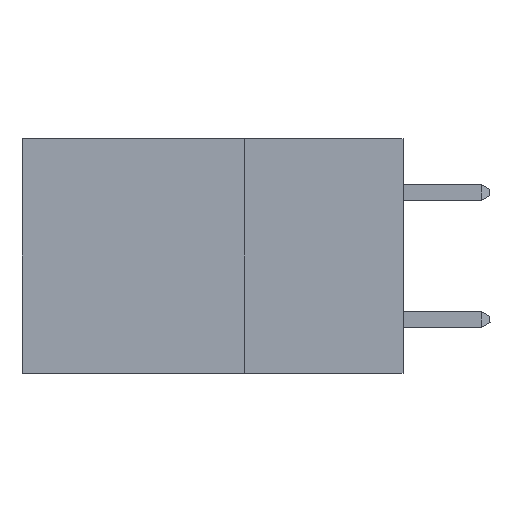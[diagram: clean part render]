
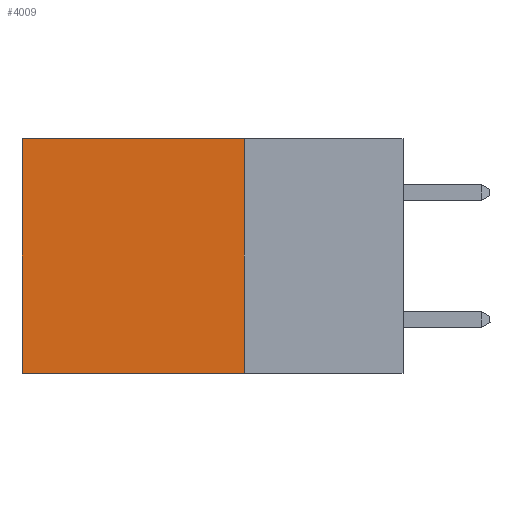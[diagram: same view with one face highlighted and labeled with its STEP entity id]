
A CAD part, left-side view. The second image highlights one B-rep face of the part: STEP entity #4009.
In plain terms, the highlighted planar face has unit normal (-1, 0, 0).
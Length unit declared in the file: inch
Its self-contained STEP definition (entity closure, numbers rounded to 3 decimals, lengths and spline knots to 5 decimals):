
#118 = VECTOR ( 'NONE', #8953, 39.37008 ) ;
#2223 = CARTESIAN_POINT ( 'NONE',  ( 0.2875, 0.25, 0. ) ) ;
#2307 = DIRECTION ( 'NONE',  ( 0., 1., 0. ) ) ;
#3486 = EDGE_LOOP ( 'NONE', ( #15040, #33119, #12994, #31197 ) ) ;
#3605 = FACE_OUTER_BOUND ( 'NONE', #3486, .T. ) ;
#3946 = VERTEX_POINT ( 'NONE', #7086 ) ;
#4009 = ADVANCED_FACE ( 'NONE', ( #3605 ), #14127, .F. ) ;
#4478 = VECTOR ( 'NONE', #2307, 39.37008 ) ;
#6650 = CARTESIAN_POINT ( 'NONE',  ( 0.2875, 0.25, 0. ) ) ;
#6898 = VECTOR ( 'NONE', #26852, 39.37008 ) ;
#7086 = CARTESIAN_POINT ( 'NONE',  ( 0.2875, 0.6, 0. ) ) ;
#7455 = LINE ( 'NONE', #6650, #19004 ) ;
#8846 = EDGE_CURVE ( 'NONE', #13015, #16911, #22549, .T. ) ;
#8953 = DIRECTION ( 'NONE',  ( 0., 0., -1. ) ) ;
#12154 = LINE ( 'NONE', #17461, #118 ) ;
#12894 = LINE ( 'NONE', #2223, #6898 ) ;
#12994 = ORIENTED_EDGE ( 'NONE', *, *, #15187, .F. ) ;
#13015 = VERTEX_POINT ( 'NONE', #30069 ) ;
#14127 = PLANE ( 'NONE',  #24519 ) ;
#15040 = ORIENTED_EDGE ( 'NONE', *, *, #25091, .T. ) ;
#15187 = EDGE_CURVE ( 'NONE', #33836, #13015, #7455, .T. ) ;
#16911 = VERTEX_POINT ( 'NONE', #22380 ) ;
#17461 = CARTESIAN_POINT ( 'NONE',  ( 0.2875, 0.6, 0. ) ) ;
#19004 = VECTOR ( 'NONE', #31744, 39.37008 ) ;
#20564 = DIRECTION ( 'NONE',  ( 1., 0., 0. ) ) ;
#22380 = CARTESIAN_POINT ( 'NONE',  ( 0.2875, 0.6, -0.37 ) ) ;
#22549 = LINE ( 'NONE', #24159, #4478 ) ;
#23369 = DIRECTION ( 'NONE',  ( 0., 0., -1. ) ) ;
#24159 = CARTESIAN_POINT ( 'NONE',  ( 0.2875, 0.25, -0.37 ) ) ;
#24519 = AXIS2_PLACEMENT_3D ( 'NONE', #28885, #20564, #23369 ) ;
#25091 = EDGE_CURVE ( 'NONE', #3946, #16911, #12154, .T. ) ;
#26852 = DIRECTION ( 'NONE',  ( 0., 1., 0. ) ) ;
#27971 = CARTESIAN_POINT ( 'NONE',  ( 0.2875, 0.25, 0. ) ) ;
#28885 = CARTESIAN_POINT ( 'NONE',  ( 0.2875, 0.25, 0. ) ) ;
#30069 = CARTESIAN_POINT ( 'NONE',  ( 0.2875, 0.25, -0.37 ) ) ;
#30996 = EDGE_CURVE ( 'NONE', #33836, #3946, #12894, .T. ) ;
#31197 = ORIENTED_EDGE ( 'NONE', *, *, #30996, .T. ) ;
#31744 = DIRECTION ( 'NONE',  ( 0., 0., -1. ) ) ;
#33119 = ORIENTED_EDGE ( 'NONE', *, *, #8846, .F. ) ;
#33836 = VERTEX_POINT ( 'NONE', #27971 ) ;
